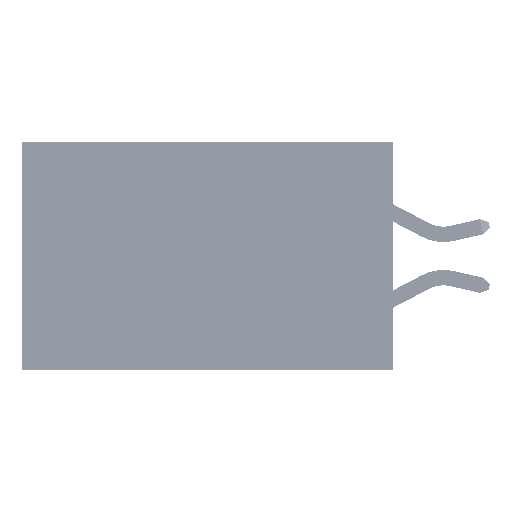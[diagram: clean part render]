
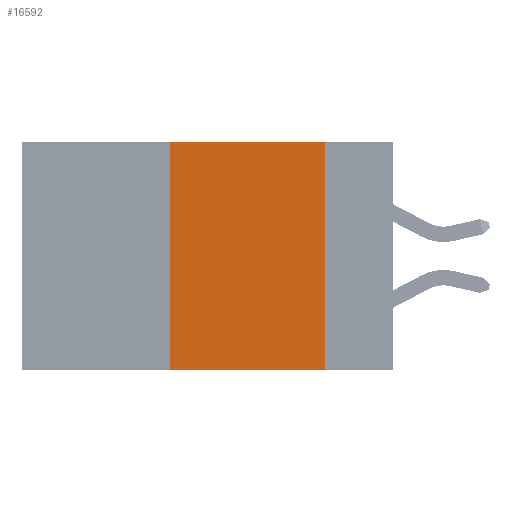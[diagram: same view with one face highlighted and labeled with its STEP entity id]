
A CAD part, left-side view. The second image highlights one B-rep face of the part: STEP entity #16592.
In plain terms, the highlighted planar face has unit normal (-1, 0, 0).
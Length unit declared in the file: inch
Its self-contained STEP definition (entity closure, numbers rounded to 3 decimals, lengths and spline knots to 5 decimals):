
#179 = VECTOR ( 'NONE', #4343, 39.37008 ) ;
#1580 = DIRECTION ( 'NONE',  ( 0., -1., 0. ) ) ;
#2907 = LINE ( 'NONE', #38695, #41988 ) ;
#3071 = CARTESIAN_POINT ( 'NONE',  ( 0., 0.11, 0. ) ) ;
#3264 = EDGE_CURVE ( 'NONE', #8655, #36465, #31176, .T. ) ;
#4343 = DIRECTION ( 'NONE',  ( 0., 0., 1. ) ) ;
#8655 = VERTEX_POINT ( 'NONE', #16990 ) ;
#9052 = CARTESIAN_POINT ( 'NONE',  ( 0., 0.36, -0.37 ) ) ;
#10522 = ORIENTED_EDGE ( 'NONE', *, *, #17669, .F. ) ;
#11680 = CARTESIAN_POINT ( 'NONE',  ( 0., 0.36, 0. ) ) ;
#12624 = ORIENTED_EDGE ( 'NONE', *, *, #3264, .F. ) ;
#13856 = AXIS2_PLACEMENT_3D ( 'NONE', #20894, #28734, #47307 ) ;
#15047 = VECTOR ( 'NONE', #1580, 39.37008 ) ;
#16465 = EDGE_CURVE ( 'NONE', #28448, #36465, #2907, .T. ) ;
#16592 = ADVANCED_FACE ( 'NONE', ( #35571 ), #40139, .F. ) ;
#16951 = DIRECTION ( 'NONE',  ( 0., -1., 0. ) ) ;
#16990 = CARTESIAN_POINT ( 'NONE',  ( 0., 0.11, 0. ) ) ;
#17669 = EDGE_CURVE ( 'NONE', #43466, #8655, #29071, .T. ) ;
#18886 = VECTOR ( 'NONE', #25735, 39.37008 ) ;
#19266 = CARTESIAN_POINT ( 'NONE',  ( 0., 0.11, -0.37 ) ) ;
#20168 = CARTESIAN_POINT ( 'NONE',  ( 0., 0.6, 0. ) ) ;
#20894 = CARTESIAN_POINT ( 'NONE',  ( 0., 0.6, 0. ) ) ;
#21659 = EDGE_LOOP ( 'NONE', ( #12624, #10522, #38803, #42309 ) ) ;
#25735 = DIRECTION ( 'NONE',  ( 0., 0., -1. ) ) ;
#28448 = VERTEX_POINT ( 'NONE', #9052 ) ;
#28734 = DIRECTION ( 'NONE',  ( 1., 0., 0. ) ) ;
#29071 = LINE ( 'NONE', #20168, #15047 ) ;
#31176 = LINE ( 'NONE', #3071, #18886 ) ;
#34079 = CARTESIAN_POINT ( 'NONE',  ( 0., 0.36, 0. ) ) ;
#35571 = FACE_OUTER_BOUND ( 'NONE', #21659, .T. ) ;
#36465 = VERTEX_POINT ( 'NONE', #19266 ) ;
#38695 = CARTESIAN_POINT ( 'NONE',  ( 0., 0.6, -0.37 ) ) ;
#38803 = ORIENTED_EDGE ( 'NONE', *, *, #40990, .F. ) ;
#40139 = PLANE ( 'NONE',  #13856 ) ;
#40990 = EDGE_CURVE ( 'NONE', #28448, #43466, #46258, .T. ) ;
#41988 = VECTOR ( 'NONE', #16951, 39.37008 ) ;
#42309 = ORIENTED_EDGE ( 'NONE', *, *, #16465, .T. ) ;
#43466 = VERTEX_POINT ( 'NONE', #34079 ) ;
#46258 = LINE ( 'NONE', #11680, #179 ) ;
#47307 = DIRECTION ( 'NONE',  ( 0., 0., -1. ) ) ;
